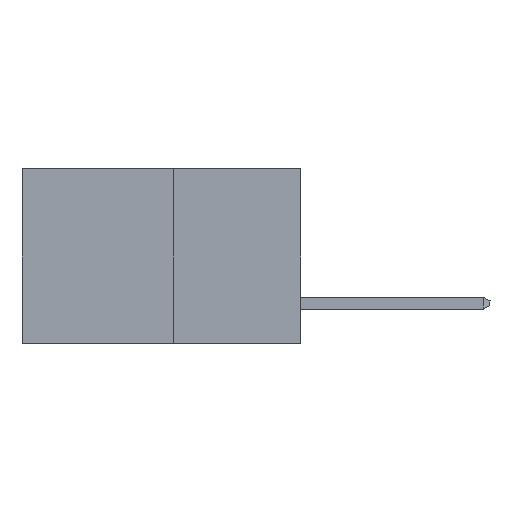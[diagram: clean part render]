
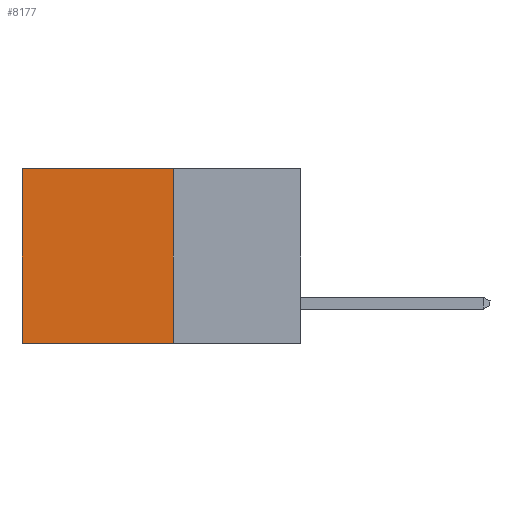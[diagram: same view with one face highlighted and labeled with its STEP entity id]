
A CAD part, left-side view. The second image highlights one B-rep face of the part: STEP entity #8177.
In plain terms, the highlighted planar face has unit normal (-1, 0, 0).
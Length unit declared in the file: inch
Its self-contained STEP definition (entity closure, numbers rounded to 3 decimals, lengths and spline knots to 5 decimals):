
#174 = DIRECTION ( 'NONE',  ( 1., 0., 0. ) ) ;
#369 = LINE ( 'NONE', #2053, #11495 ) ;
#564 = EDGE_LOOP ( 'NONE', ( #7235, #6175, #7276, #3731 ) ) ;
#632 = LINE ( 'NONE', #7086, #2776 ) ;
#1045 = EDGE_CURVE ( 'NONE', #6137, #11143, #4409, .T. ) ;
#1846 = CARTESIAN_POINT ( 'NONE',  ( 0.277, 0.27, -0.37 ) ) ;
#2004 = CARTESIAN_POINT ( 'NONE',  ( 0.277, 0.27, -0.37 ) ) ;
#2025 = CARTESIAN_POINT ( 'NONE',  ( 0.277, 0.59, 0. ) ) ;
#2053 = CARTESIAN_POINT ( 'NONE',  ( 0.277, 0.27, -0.37 ) ) ;
#2531 = VECTOR ( 'NONE', #8038, 39.37008 ) ;
#2776 = VECTOR ( 'NONE', #4423, 39.37008 ) ;
#3307 = CARTESIAN_POINT ( 'NONE',  ( 0.277, 0.27, 0. ) ) ;
#3388 = VERTEX_POINT ( 'NONE', #7846 ) ;
#3731 = ORIENTED_EDGE ( 'NONE', *, *, #6387, .T. ) ;
#4409 = LINE ( 'NONE', #1846, #2531 ) ;
#4423 = DIRECTION ( 'NONE',  ( 0., 0., -1. ) ) ;
#4735 = PLANE ( 'NONE',  #7619 ) ;
#5475 = CARTESIAN_POINT ( 'NONE',  ( 0.277, 0.27, 0. ) ) ;
#6137 = VERTEX_POINT ( 'NONE', #3307 ) ;
#6175 = ORIENTED_EDGE ( 'NONE', *, *, #10089, .F. ) ;
#6341 = FACE_OUTER_BOUND ( 'NONE', #564, .T. ) ;
#6387 = EDGE_CURVE ( 'NONE', #6137, #7500, #9388, .T. ) ;
#6532 = DIRECTION ( 'NONE',  ( 0., 0., -1. ) ) ;
#6621 = DIRECTION ( 'NONE',  ( 0., 1., 0. ) ) ;
#6960 = VECTOR ( 'NONE', #7280, 39.37008 ) ;
#7086 = CARTESIAN_POINT ( 'NONE',  ( 0.277, 0.59, -0.37 ) ) ;
#7235 = ORIENTED_EDGE ( 'NONE', *, *, #10428, .T. ) ;
#7276 = ORIENTED_EDGE ( 'NONE', *, *, #1045, .F. ) ;
#7280 = DIRECTION ( 'NONE',  ( 0., 1., 0. ) ) ;
#7500 = VERTEX_POINT ( 'NONE', #2025 ) ;
#7619 = AXIS2_PLACEMENT_3D ( 'NONE', #10981, #174, #6532 ) ;
#7846 = CARTESIAN_POINT ( 'NONE',  ( 0.277, 0.59, -0.37 ) ) ;
#8038 = DIRECTION ( 'NONE',  ( 0., 0., -1. ) ) ;
#8177 = ADVANCED_FACE ( 'NONE', ( #6341 ), #4735, .F. ) ;
#9388 = LINE ( 'NONE', #5475, #6960 ) ;
#10089 = EDGE_CURVE ( 'NONE', #11143, #3388, #369, .T. ) ;
#10428 = EDGE_CURVE ( 'NONE', #7500, #3388, #632, .T. ) ;
#10981 = CARTESIAN_POINT ( 'NONE',  ( 0.277, 0.27, -0.37 ) ) ;
#11143 = VERTEX_POINT ( 'NONE', #2004 ) ;
#11495 = VECTOR ( 'NONE', #6621, 39.37008 ) ;
